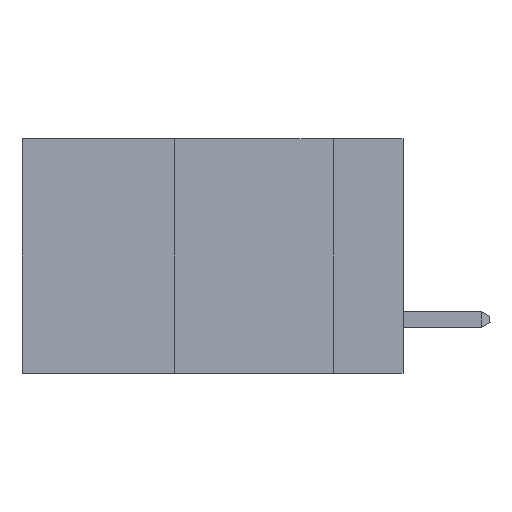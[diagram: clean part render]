
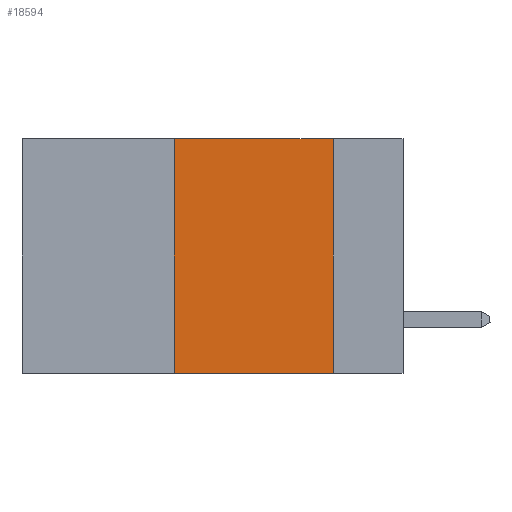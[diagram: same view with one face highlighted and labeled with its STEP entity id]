
A CAD part, left-side view. The second image highlights one B-rep face of the part: STEP entity #18594.
In plain terms, the highlighted planar face has unit normal (-1, 0, 0).
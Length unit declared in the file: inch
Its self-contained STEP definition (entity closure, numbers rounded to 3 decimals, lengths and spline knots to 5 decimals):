
#403 = LINE ( 'NONE', #20254, #6274 ) ;
#1267 = VECTOR ( 'NONE', #18693, 39.37008 ) ;
#1404 = ORIENTED_EDGE ( 'NONE', *, *, #6220, .F. ) ;
#1500 = FACE_OUTER_BOUND ( 'NONE', #19183, .T. ) ;
#2405 = VERTEX_POINT ( 'NONE', #2848 ) ;
#2848 = CARTESIAN_POINT ( 'NONE',  ( 0., 0.11, 0. ) ) ;
#2953 = VECTOR ( 'NONE', #26780, 39.37008 ) ;
#4123 = LINE ( 'NONE', #13959, #20235 ) ;
#4441 = EDGE_CURVE ( 'NONE', #17262, #18754, #8446, .T. ) ;
#4786 = EDGE_CURVE ( 'NONE', #17262, #6377, #11617, .T. ) ;
#6220 = EDGE_CURVE ( 'NONE', #6377, #2405, #4123, .T. ) ;
#6274 = VECTOR ( 'NONE', #18440, 39.37008 ) ;
#6327 = CARTESIAN_POINT ( 'NONE',  ( 0., 0.6, 0. ) ) ;
#6377 = VERTEX_POINT ( 'NONE', #10350 ) ;
#6405 = ORIENTED_EDGE ( 'NONE', *, *, #4786, .F. ) ;
#8446 = LINE ( 'NONE', #20265, #2953 ) ;
#9459 = DIRECTION ( 'NONE',  ( 0., -1., 0. ) ) ;
#10350 = CARTESIAN_POINT ( 'NONE',  ( 0., 0.36, 0. ) ) ;
#10541 = DIRECTION ( 'NONE',  ( 0., 0., -1. ) ) ;
#10975 = CARTESIAN_POINT ( 'NONE',  ( 0., 0.11, -0.37 ) ) ;
#11617 = LINE ( 'NONE', #16423, #1267 ) ;
#13722 = AXIS2_PLACEMENT_3D ( 'NONE', #6327, #16390, #10541 ) ;
#13959 = CARTESIAN_POINT ( 'NONE',  ( 0., 0.6, 0. ) ) ;
#16390 = DIRECTION ( 'NONE',  ( 1., 0., 0. ) ) ;
#16423 = CARTESIAN_POINT ( 'NONE',  ( 0., 0.36, 0. ) ) ;
#16749 = PLANE ( 'NONE',  #13722 ) ;
#17037 = ORIENTED_EDGE ( 'NONE', *, *, #20938, .F. ) ;
#17262 = VERTEX_POINT ( 'NONE', #20193 ) ;
#18440 = DIRECTION ( 'NONE',  ( 0., 0., -1. ) ) ;
#18594 = ADVANCED_FACE ( 'NONE', ( #1500 ), #16749, .F. ) ;
#18693 = DIRECTION ( 'NONE',  ( 0., 0., 1. ) ) ;
#18754 = VERTEX_POINT ( 'NONE', #10975 ) ;
#19119 = ORIENTED_EDGE ( 'NONE', *, *, #4441, .T. ) ;
#19183 = EDGE_LOOP ( 'NONE', ( #17037, #1404, #6405, #19119 ) ) ;
#20193 = CARTESIAN_POINT ( 'NONE',  ( 0., 0.36, -0.37 ) ) ;
#20235 = VECTOR ( 'NONE', #9459, 39.37008 ) ;
#20254 = CARTESIAN_POINT ( 'NONE',  ( 0., 0.11, 0. ) ) ;
#20265 = CARTESIAN_POINT ( 'NONE',  ( 0., 0.6, -0.37 ) ) ;
#20938 = EDGE_CURVE ( 'NONE', #2405, #18754, #403, .T. ) ;
#26780 = DIRECTION ( 'NONE',  ( 0., -1., 0. ) ) ;
